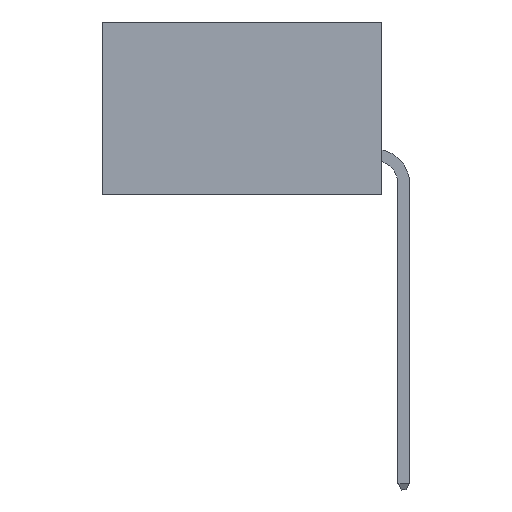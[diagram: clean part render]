
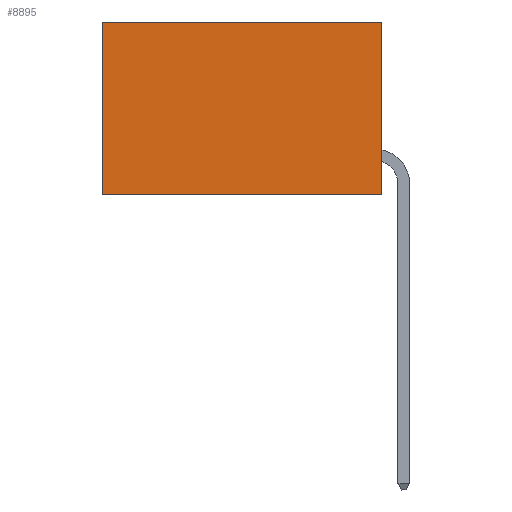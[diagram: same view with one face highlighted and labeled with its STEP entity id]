
A CAD part, left-side view. The second image highlights one B-rep face of the part: STEP entity #8895.
In plain terms, the highlighted planar face has unit normal (-1, 0, 0).
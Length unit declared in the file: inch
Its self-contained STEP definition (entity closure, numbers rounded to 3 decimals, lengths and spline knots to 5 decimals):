
#214 = LINE ( 'NONE', #2241, #5152 ) ;
#240 = ORIENTED_EDGE ( 'NONE', *, *, #10367, .T. ) ;
#252 = DIRECTION ( 'NONE',  ( 0., 1., 0. ) ) ;
#428 = VERTEX_POINT ( 'NONE', #10363 ) ;
#982 = PLANE ( 'NONE',  #2233 ) ;
#1034 = VECTOR ( 'NONE', #252, 39.37008 ) ;
#1111 = ORIENTED_EDGE ( 'NONE', *, *, #9061, .T. ) ;
#1160 = ORIENTED_EDGE ( 'NONE', *, *, #5654, .F. ) ;
#1685 = DIRECTION ( 'NONE',  ( 0., 0., -1. ) ) ;
#1744 = FACE_OUTER_BOUND ( 'NONE', #4246, .T. ) ;
#2023 = CARTESIAN_POINT ( 'NONE',  ( 0.2875, 0.6, 0. ) ) ;
#2233 = AXIS2_PLACEMENT_3D ( 'NONE', #9093, #7464, #3418 ) ;
#2241 = CARTESIAN_POINT ( 'NONE',  ( 0.2875, 0., 0. ) ) ;
#2368 = LINE ( 'NONE', #8960, #8647 ) ;
#3051 = DIRECTION ( 'NONE',  ( 0., 1., 0. ) ) ;
#3418 = DIRECTION ( 'NONE',  ( 0., 0., -1. ) ) ;
#3572 = VERTEX_POINT ( 'NONE', #10415 ) ;
#4246 = EDGE_LOOP ( 'NONE', ( #1111, #1160, #9929, #240 ) ) ;
#4359 = VECTOR ( 'NONE', #7534, 39.37008 ) ;
#4955 = CARTESIAN_POINT ( 'NONE',  ( 0.2875, 0., 0. ) ) ;
#5140 = VERTEX_POINT ( 'NONE', #7309 ) ;
#5152 = VECTOR ( 'NONE', #3051, 39.37008 ) ;
#5654 = EDGE_CURVE ( 'NONE', #428, #5140, #10217, .T. ) ;
#7309 = CARTESIAN_POINT ( 'NONE',  ( 0.2875, 0.6, -0.37 ) ) ;
#7464 = DIRECTION ( 'NONE',  ( 1., 0., 0. ) ) ;
#7534 = DIRECTION ( 'NONE',  ( 0., 0., -1. ) ) ;
#8647 = VECTOR ( 'NONE', #1685, 39.37008 ) ;
#8895 = ADVANCED_FACE ( 'NONE', ( #1744 ), #982, .F. ) ;
#8960 = CARTESIAN_POINT ( 'NONE',  ( 0.2875, 0., 0. ) ) ;
#9061 = EDGE_CURVE ( 'NONE', #3572, #5140, #10404, .T. ) ;
#9093 = CARTESIAN_POINT ( 'NONE',  ( 0.2875, 0., 0. ) ) ;
#9489 = EDGE_CURVE ( 'NONE', #9859, #428, #2368, .T. ) ;
#9763 = CARTESIAN_POINT ( 'NONE',  ( 0.2875, 0., -0.37 ) ) ;
#9859 = VERTEX_POINT ( 'NONE', #4955 ) ;
#9929 = ORIENTED_EDGE ( 'NONE', *, *, #9489, .F. ) ;
#10217 = LINE ( 'NONE', #9763, #1034 ) ;
#10363 = CARTESIAN_POINT ( 'NONE',  ( 0.2875, 0., -0.37 ) ) ;
#10367 = EDGE_CURVE ( 'NONE', #9859, #3572, #214, .T. ) ;
#10404 = LINE ( 'NONE', #2023, #4359 ) ;
#10415 = CARTESIAN_POINT ( 'NONE',  ( 0.2875, 0.6, 0. ) ) ;
